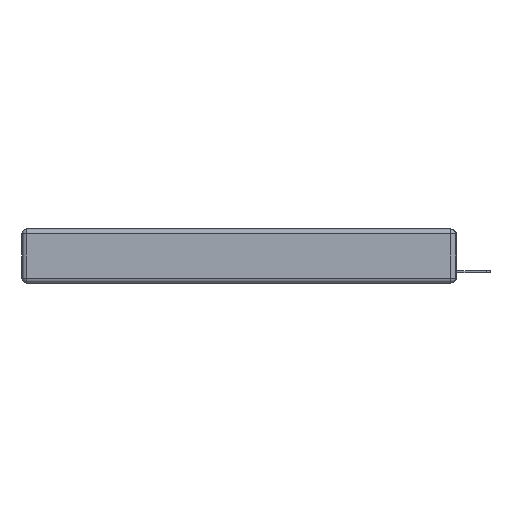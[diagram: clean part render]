
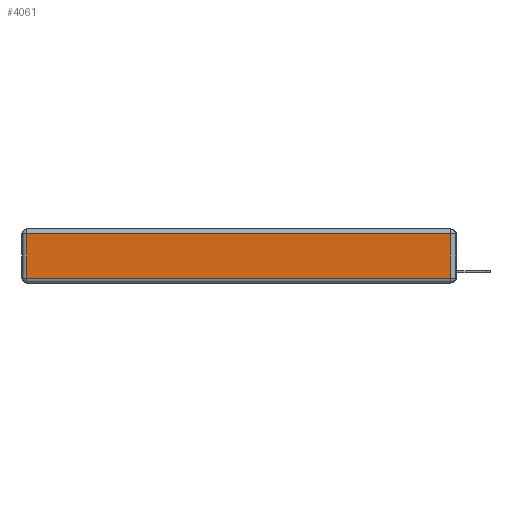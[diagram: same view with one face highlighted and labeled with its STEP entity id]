
A CAD part, left-side view. The second image highlights one B-rep face of the part: STEP entity #4061.
In plain terms, the highlighted planar face has unit normal (-1, 0, 0).
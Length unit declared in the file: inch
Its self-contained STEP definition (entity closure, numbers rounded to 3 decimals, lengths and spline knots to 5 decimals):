
#565 = CARTESIAN_POINT ( 'NONE',  ( 0., 2.75, -0.03 ) ) ;
#1020 = ORIENTED_EDGE ( 'NONE', *, *, #3785, .T. ) ;
#1385 = EDGE_CURVE ( 'NONE', #14728, #15418, #22196, .T. ) ;
#2229 = DIRECTION ( 'NONE',  ( 0., 0., 1. ) ) ;
#2373 = DIRECTION ( 'NONE',  ( 0., 1., 0. ) ) ;
#2544 = DIRECTION ( 'NONE',  ( 0., 0., -1. ) ) ;
#2643 = EDGE_LOOP ( 'NONE', ( #5985, #1020, #3486, #2746 ) ) ;
#2746 = ORIENTED_EDGE ( 'NONE', *, *, #1385, .T. ) ;
#3486 = ORIENTED_EDGE ( 'NONE', *, *, #24636, .T. ) ;
#3727 = LINE ( 'NONE', #14089, #18875 ) ;
#3747 = VERTEX_POINT ( 'NONE', #23546 ) ;
#3785 = EDGE_CURVE ( 'NONE', #10187, #3747, #13420, .T. ) ;
#3998 = CARTESIAN_POINT ( 'NONE',  ( 0., 2.72, -0.343 ) ) ;
#4061 = ADVANCED_FACE ( 'NONE', ( #25508 ), #21599, .T. ) ;
#4126 = CARTESIAN_POINT ( 'NONE',  ( 0., 2.72, -0.313 ) ) ;
#5742 = CARTESIAN_POINT ( 'NONE',  ( 0., 0., -0.343 ) ) ;
#5985 = ORIENTED_EDGE ( 'NONE', *, *, #21315, .T. ) ;
#9680 = DIRECTION ( 'NONE',  ( -1., 0., 0. ) ) ;
#10187 = VERTEX_POINT ( 'NONE', #14162 ) ;
#11476 = DIRECTION ( 'NONE',  ( 0., 0., 1. ) ) ;
#13420 = LINE ( 'NONE', #16349, #14659 ) ;
#14055 = LINE ( 'NONE', #565, #21159 ) ;
#14089 = CARTESIAN_POINT ( 'NONE',  ( 0., 0., -0.313 ) ) ;
#14162 = CARTESIAN_POINT ( 'NONE',  ( 0., 0.03, -0.313 ) ) ;
#14659 = VECTOR ( 'NONE', #2229, 39.37008 ) ;
#14728 = VERTEX_POINT ( 'NONE', #20620 ) ;
#15418 = VERTEX_POINT ( 'NONE', #4126 ) ;
#15448 = AXIS2_PLACEMENT_3D ( 'NONE', #5742, #9680, #11476 ) ;
#16349 = CARTESIAN_POINT ( 'NONE',  ( 0., 0.03, -0.343 ) ) ;
#18875 = VECTOR ( 'NONE', #23955, 39.37008 ) ;
#20620 = CARTESIAN_POINT ( 'NONE',  ( 0., 2.72, -0.03 ) ) ;
#21159 = VECTOR ( 'NONE', #2373, 39.37008 ) ;
#21315 = EDGE_CURVE ( 'NONE', #15418, #10187, #3727, .T. ) ;
#21599 = PLANE ( 'NONE',  #15448 ) ;
#22196 = LINE ( 'NONE', #3998, #24369 ) ;
#23546 = CARTESIAN_POINT ( 'NONE',  ( 0., 0.03, -0.03 ) ) ;
#23955 = DIRECTION ( 'NONE',  ( 0., -1., 0. ) ) ;
#24369 = VECTOR ( 'NONE', #2544, 39.37008 ) ;
#24636 = EDGE_CURVE ( 'NONE', #3747, #14728, #14055, .T. ) ;
#25508 = FACE_OUTER_BOUND ( 'NONE', #2643, .T. ) ;
